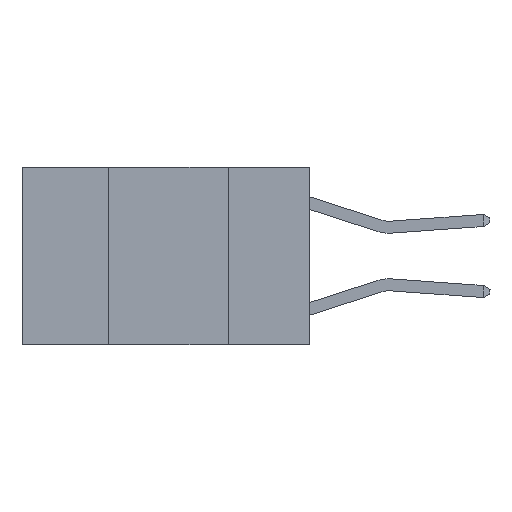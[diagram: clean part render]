
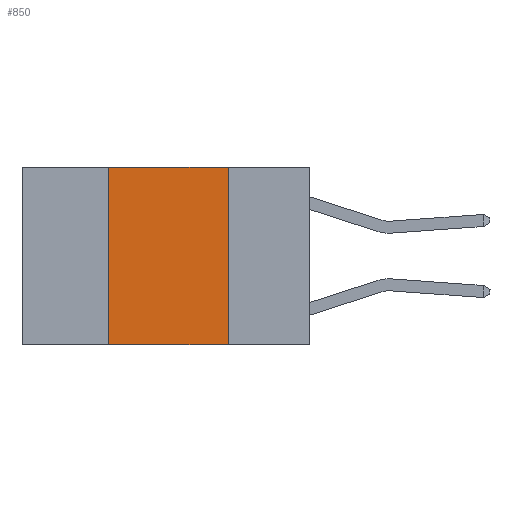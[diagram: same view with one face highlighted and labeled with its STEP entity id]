
A CAD part, left-side view. The second image highlights one B-rep face of the part: STEP entity #850.
In plain terms, the highlighted planar face has unit normal (-1, 0, 0).
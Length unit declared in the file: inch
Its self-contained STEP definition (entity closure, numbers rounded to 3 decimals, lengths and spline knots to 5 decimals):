
#686 = FACE_OUTER_BOUND ( 'NONE', #2436, .T. ) ;
#850 = ADVANCED_FACE ( 'NONE', ( #686 ), #2467, .F. ) ;
#2436 = EDGE_LOOP ( 'NONE', ( #8672, #10799, #5587, #9673 ) ) ;
#2467 = PLANE ( 'NONE',  #12776 ) ;
#2492 = DIRECTION ( 'NONE',  ( 0., 0., -1. ) ) ;
#2506 = VERTEX_POINT ( 'NONE', #9509 ) ;
#2773 = CARTESIAN_POINT ( 'NONE',  ( 0., 0.42, 0. ) ) ;
#2789 = VERTEX_POINT ( 'NONE', #10008 ) ;
#3049 = CARTESIAN_POINT ( 'NONE',  ( 0., 0.42, 0. ) ) ;
#3735 = VECTOR ( 'NONE', #9972, 39.37008 ) ;
#4295 = VECTOR ( 'NONE', #4357, 39.37008 ) ;
#4357 = DIRECTION ( 'NONE',  ( 0., -1., 0. ) ) ;
#4725 = EDGE_CURVE ( 'NONE', #2506, #7796, #13505, .T. ) ;
#5587 = ORIENTED_EDGE ( 'NONE', *, *, #4725, .F. ) ;
#6194 = VECTOR ( 'NONE', #8704, 39.37008 ) ;
#6619 = EDGE_CURVE ( 'NONE', #7796, #2789, #9863, .T. ) ;
#7344 = CARTESIAN_POINT ( 'NONE',  ( 0., 0.6, 0. ) ) ;
#7686 = CARTESIAN_POINT ( 'NONE',  ( 0., 0.6, -0.37 ) ) ;
#7796 = VERTEX_POINT ( 'NONE', #3049 ) ;
#8478 = EDGE_CURVE ( 'NONE', #2789, #8806, #9640, .T. ) ;
#8672 = ORIENTED_EDGE ( 'NONE', *, *, #8478, .F. ) ;
#8704 = DIRECTION ( 'NONE',  ( 0., -1., 0. ) ) ;
#8806 = VERTEX_POINT ( 'NONE', #12641 ) ;
#8918 = CARTESIAN_POINT ( 'NONE',  ( 0., 0.17, 0. ) ) ;
#8959 = LINE ( 'NONE', #7686, #6194 ) ;
#9044 = DIRECTION ( 'NONE',  ( 0., 0., 1. ) ) ;
#9509 = CARTESIAN_POINT ( 'NONE',  ( 0., 0.42, -0.37 ) ) ;
#9637 = EDGE_CURVE ( 'NONE', #2506, #8806, #8959, .T. ) ;
#9640 = LINE ( 'NONE', #8918, #3735 ) ;
#9673 = ORIENTED_EDGE ( 'NONE', *, *, #9637, .T. ) ;
#9707 = DIRECTION ( 'NONE',  ( 1., 0., 0. ) ) ;
#9863 = LINE ( 'NONE', #10616, #4295 ) ;
#9972 = DIRECTION ( 'NONE',  ( 0., 0., -1. ) ) ;
#10008 = CARTESIAN_POINT ( 'NONE',  ( 0., 0.17, 0. ) ) ;
#10616 = CARTESIAN_POINT ( 'NONE',  ( 0., 0.6, 0. ) ) ;
#10709 = VECTOR ( 'NONE', #9044, 39.37008 ) ;
#10799 = ORIENTED_EDGE ( 'NONE', *, *, #6619, .F. ) ;
#12641 = CARTESIAN_POINT ( 'NONE',  ( 0., 0.17, -0.37 ) ) ;
#12776 = AXIS2_PLACEMENT_3D ( 'NONE', #7344, #9707, #2492 ) ;
#13505 = LINE ( 'NONE', #2773, #10709 ) ;
